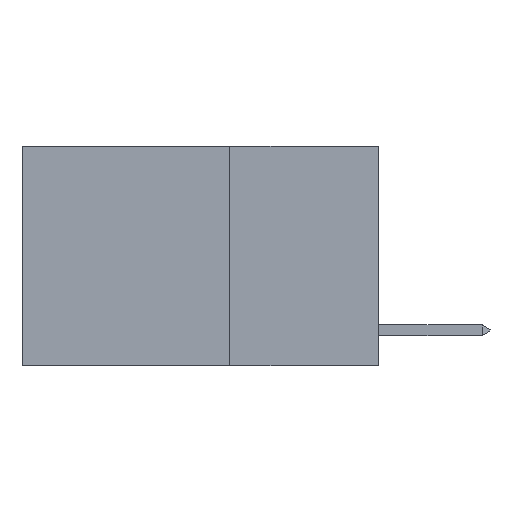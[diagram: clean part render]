
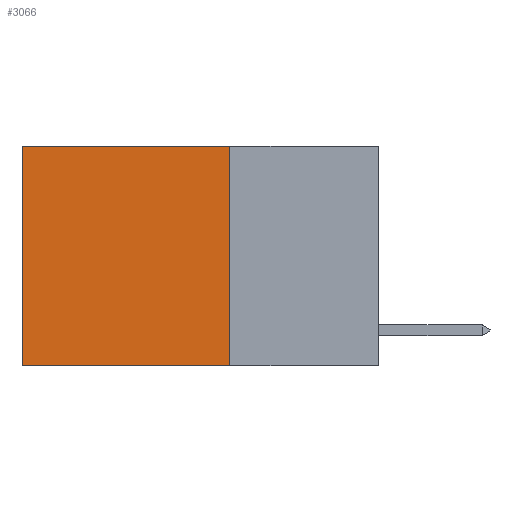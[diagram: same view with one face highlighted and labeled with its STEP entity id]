
A CAD part, left-side view. The second image highlights one B-rep face of the part: STEP entity #3066.
In plain terms, the highlighted planar face has unit normal (-1, 0, 0).
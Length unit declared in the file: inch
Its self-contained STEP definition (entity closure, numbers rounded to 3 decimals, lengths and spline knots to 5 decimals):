
#263 = ORIENTED_EDGE ( 'NONE', *, *, #5156, .F. ) ;
#387 = CARTESIAN_POINT ( 'NONE',  ( 0.2625, 0.25, 0. ) ) ;
#824 = VERTEX_POINT ( 'NONE', #1863 ) ;
#892 = CARTESIAN_POINT ( 'NONE',  ( 0.2625, 0.25, 0. ) ) ;
#1308 = LINE ( 'NONE', #9333, #2648 ) ;
#1535 = PLANE ( 'NONE',  #3230 ) ;
#1609 = FACE_OUTER_BOUND ( 'NONE', #4782, .T. ) ;
#1672 = ORIENTED_EDGE ( 'NONE', *, *, #10943, .T. ) ;
#1863 = CARTESIAN_POINT ( 'NONE',  ( 0.2625, 0.6, -0.37 ) ) ;
#2648 = VECTOR ( 'NONE', #9213, 39.37008 ) ;
#2875 = ORIENTED_EDGE ( 'NONE', *, *, #5641, .F. ) ;
#2889 = CARTESIAN_POINT ( 'NONE',  ( 0.2625, 0.25, 0. ) ) ;
#3066 = ADVANCED_FACE ( 'NONE', ( #1609 ), #1535, .F. ) ;
#3230 = AXIS2_PLACEMENT_3D ( 'NONE', #892, #4847, #7668 ) ;
#4012 = LINE ( 'NONE', #10562, #10237 ) ;
#4061 = VERTEX_POINT ( 'NONE', #4911 ) ;
#4274 = EDGE_CURVE ( 'NONE', #4061, #824, #4012, .T. ) ;
#4782 = EDGE_LOOP ( 'NONE', ( #5745, #263, #2875, #1672 ) ) ;
#4847 = DIRECTION ( 'NONE',  ( 1., 0., 0. ) ) ;
#4911 = CARTESIAN_POINT ( 'NONE',  ( 0.2625, 0.6, 0. ) ) ;
#4970 = CARTESIAN_POINT ( 'NONE',  ( 0.2625, 0.25, -0.37 ) ) ;
#5156 = EDGE_CURVE ( 'NONE', #9694, #824, #8060, .T. ) ;
#5641 = EDGE_CURVE ( 'NONE', #7049, #9694, #5863, .T. ) ;
#5707 = DIRECTION ( 'NONE',  ( 0., 0., -1. ) ) ;
#5745 = ORIENTED_EDGE ( 'NONE', *, *, #4274, .T. ) ;
#5863 = LINE ( 'NONE', #2889, #7452 ) ;
#7049 = VERTEX_POINT ( 'NONE', #387 ) ;
#7452 = VECTOR ( 'NONE', #5707, 39.37008 ) ;
#7668 = DIRECTION ( 'NONE',  ( 0., 0., -1. ) ) ;
#7715 = DIRECTION ( 'NONE',  ( 0., 0., -1. ) ) ;
#7740 = VECTOR ( 'NONE', #11718, 39.37008 ) ;
#8060 = LINE ( 'NONE', #11671, #7740 ) ;
#9213 = DIRECTION ( 'NONE',  ( 0., 1., 0. ) ) ;
#9333 = CARTESIAN_POINT ( 'NONE',  ( 0.2625, 0.25, 0. ) ) ;
#9694 = VERTEX_POINT ( 'NONE', #4970 ) ;
#10237 = VECTOR ( 'NONE', #7715, 39.37008 ) ;
#10562 = CARTESIAN_POINT ( 'NONE',  ( 0.2625, 0.6, 0. ) ) ;
#10943 = EDGE_CURVE ( 'NONE', #7049, #4061, #1308, .T. ) ;
#11671 = CARTESIAN_POINT ( 'NONE',  ( 0.2625, 0.25, -0.37 ) ) ;
#11718 = DIRECTION ( 'NONE',  ( 0., 1., 0. ) ) ;
